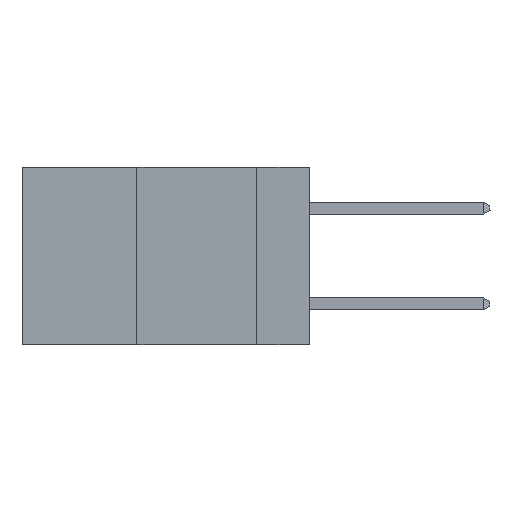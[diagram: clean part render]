
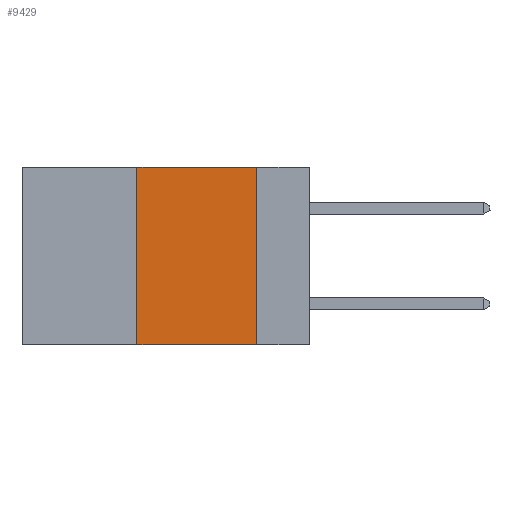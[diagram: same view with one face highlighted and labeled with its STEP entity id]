
A CAD part, left-side view. The second image highlights one B-rep face of the part: STEP entity #9429.
In plain terms, the highlighted planar face has unit normal (-1, 0, 0).
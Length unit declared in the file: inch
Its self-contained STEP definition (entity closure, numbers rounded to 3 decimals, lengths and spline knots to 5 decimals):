
#794 = VERTEX_POINT ( 'NONE', #16297 ) ;
#837 = EDGE_CURVE ( 'NONE', #9021, #4740, #14158, .T. ) ;
#1121 = CARTESIAN_POINT ( 'NONE',  ( 0., 0.36, 0. ) ) ;
#1987 = LINE ( 'NONE', #22439, #11909 ) ;
#3089 = VECTOR ( 'NONE', #22014, 39.37008 ) ;
#3405 = LINE ( 'NONE', #1121, #4360 ) ;
#3734 = DIRECTION ( 'NONE',  ( 0., -1., 0. ) ) ;
#4360 = VECTOR ( 'NONE', #9281, 39.37008 ) ;
#4520 = ORIENTED_EDGE ( 'NONE', *, *, #22881, .F. ) ;
#4740 = VERTEX_POINT ( 'NONE', #21699 ) ;
#5391 = EDGE_LOOP ( 'NONE', ( #4520, #24282, #22587, #8429 ) ) ;
#6112 = CARTESIAN_POINT ( 'NONE',  ( 0., 0.6, -0.37 ) ) ;
#7559 = VECTOR ( 'NONE', #3734, 39.37008 ) ;
#8429 = ORIENTED_EDGE ( 'NONE', *, *, #12886, .T. ) ;
#9021 = VERTEX_POINT ( 'NONE', #20475 ) ;
#9281 = DIRECTION ( 'NONE',  ( 0., 0., 1. ) ) ;
#9429 = ADVANCED_FACE ( 'NONE', ( #15931 ), #26392, .F. ) ;
#11862 = LINE ( 'NONE', #6112, #3089 ) ;
#11909 = VECTOR ( 'NONE', #24308, 39.37008 ) ;
#12174 = DIRECTION ( 'NONE',  ( 0., 0., -1. ) ) ;
#12886 = EDGE_CURVE ( 'NONE', #14264, #794, #11862, .T. ) ;
#13024 = EDGE_CURVE ( 'NONE', #14264, #9021, #3405, .T. ) ;
#14158 = LINE ( 'NONE', #24169, #7559 ) ;
#14264 = VERTEX_POINT ( 'NONE', #20281 ) ;
#15931 = FACE_OUTER_BOUND ( 'NONE', #5391, .T. ) ;
#16297 = CARTESIAN_POINT ( 'NONE',  ( 0., 0.11, -0.37 ) ) ;
#20281 = CARTESIAN_POINT ( 'NONE',  ( 0., 0.36, -0.37 ) ) ;
#20475 = CARTESIAN_POINT ( 'NONE',  ( 0., 0.36, 0. ) ) ;
#21699 = CARTESIAN_POINT ( 'NONE',  ( 0., 0.11, 0. ) ) ;
#21733 = AXIS2_PLACEMENT_3D ( 'NONE', #24188, #24575, #12174 ) ;
#22014 = DIRECTION ( 'NONE',  ( 0., -1., 0. ) ) ;
#22439 = CARTESIAN_POINT ( 'NONE',  ( 0., 0.11, 0. ) ) ;
#22587 = ORIENTED_EDGE ( 'NONE', *, *, #13024, .F. ) ;
#22881 = EDGE_CURVE ( 'NONE', #4740, #794, #1987, .T. ) ;
#24169 = CARTESIAN_POINT ( 'NONE',  ( 0., 0.6, 0. ) ) ;
#24188 = CARTESIAN_POINT ( 'NONE',  ( 0., 0.6, 0. ) ) ;
#24282 = ORIENTED_EDGE ( 'NONE', *, *, #837, .F. ) ;
#24308 = DIRECTION ( 'NONE',  ( 0., 0., -1. ) ) ;
#24575 = DIRECTION ( 'NONE',  ( 1., 0., 0. ) ) ;
#26392 = PLANE ( 'NONE',  #21733 ) ;
